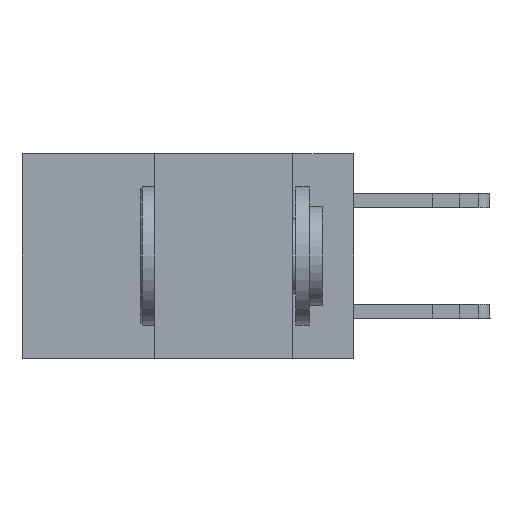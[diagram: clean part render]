
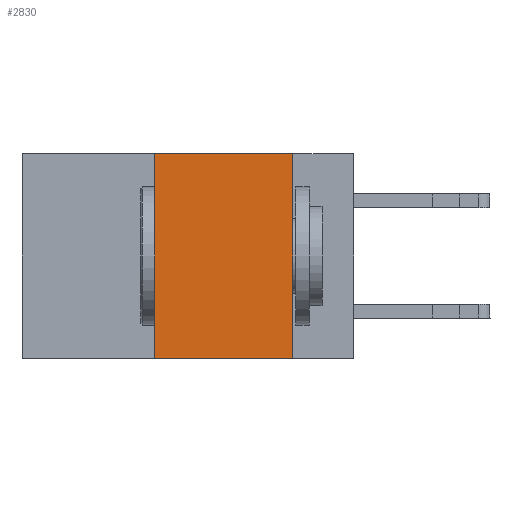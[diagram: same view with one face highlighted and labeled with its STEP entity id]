
A CAD part, left-side view. The second image highlights one B-rep face of the part: STEP entity #2830.
In plain terms, the highlighted planar face has unit normal (-1, 0, 0).
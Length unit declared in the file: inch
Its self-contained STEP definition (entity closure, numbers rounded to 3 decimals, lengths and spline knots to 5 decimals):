
#465 = DIRECTION ( 'NONE',  ( 0., 0., 1. ) ) ;
#1585 = LINE ( 'NONE', #6377, #13972 ) ;
#1826 = EDGE_CURVE ( 'NONE', #8082, #3383, #12513, .T. ) ;
#2120 = CARTESIAN_POINT ( 'NONE',  ( 0., 0.11, -0.37 ) ) ;
#2216 = FACE_OUTER_BOUND ( 'NONE', #5645, .T. ) ;
#2830 = ADVANCED_FACE ( 'NONE', ( #2216 ), #16677, .F. ) ;
#2837 = CARTESIAN_POINT ( 'NONE',  ( 0., 0.36, -0.37 ) ) ;
#3383 = VERTEX_POINT ( 'NONE', #16611 ) ;
#4227 = VERTEX_POINT ( 'NONE', #2837 ) ;
#4264 = VECTOR ( 'NONE', #7695, 39.37008 ) ;
#4555 = VECTOR ( 'NONE', #465, 39.37008 ) ;
#5645 = EDGE_LOOP ( 'NONE', ( #16928, #16864, #11952, #11885 ) ) ;
#6377 = CARTESIAN_POINT ( 'NONE',  ( 0., 0.6, -0.37 ) ) ;
#7304 = CARTESIAN_POINT ( 'NONE',  ( 0., 0.11, 0. ) ) ;
#7695 = DIRECTION ( 'NONE',  ( 0., -1., 0. ) ) ;
#7908 = CARTESIAN_POINT ( 'NONE',  ( 0., 0.6, 0. ) ) ;
#8082 = VERTEX_POINT ( 'NONE', #9760 ) ;
#8088 = AXIS2_PLACEMENT_3D ( 'NONE', #17485, #16309, #16307 ) ;
#8349 = CARTESIAN_POINT ( 'NONE',  ( 0., 0.36, 0. ) ) ;
#9760 = CARTESIAN_POINT ( 'NONE',  ( 0., 0.36, 0. ) ) ;
#11633 = VECTOR ( 'NONE', #18050, 39.37008 ) ;
#11885 = ORIENTED_EDGE ( 'NONE', *, *, #14527, .T. ) ;
#11952 = ORIENTED_EDGE ( 'NONE', *, *, #19634, .F. ) ;
#12513 = LINE ( 'NONE', #7908, #4264 ) ;
#13972 = VECTOR ( 'NONE', #17117, 39.37008 ) ;
#14527 = EDGE_CURVE ( 'NONE', #4227, #16606, #1585, .T. ) ;
#14701 = LINE ( 'NONE', #7304, #11633 ) ;
#16307 = DIRECTION ( 'NONE',  ( 0., 0., -1. ) ) ;
#16309 = DIRECTION ( 'NONE',  ( 1., 0., 0. ) ) ;
#16606 = VERTEX_POINT ( 'NONE', #2120 ) ;
#16611 = CARTESIAN_POINT ( 'NONE',  ( 0., 0.11, 0. ) ) ;
#16677 = PLANE ( 'NONE',  #8088 ) ;
#16816 = LINE ( 'NONE', #8349, #4555 ) ;
#16864 = ORIENTED_EDGE ( 'NONE', *, *, #1826, .F. ) ;
#16928 = ORIENTED_EDGE ( 'NONE', *, *, #18626, .F. ) ;
#17117 = DIRECTION ( 'NONE',  ( 0., -1., 0. ) ) ;
#17485 = CARTESIAN_POINT ( 'NONE',  ( 0., 0.6, 0. ) ) ;
#18050 = DIRECTION ( 'NONE',  ( 0., 0., -1. ) ) ;
#18626 = EDGE_CURVE ( 'NONE', #3383, #16606, #14701, .T. ) ;
#19634 = EDGE_CURVE ( 'NONE', #4227, #8082, #16816, .T. ) ;
